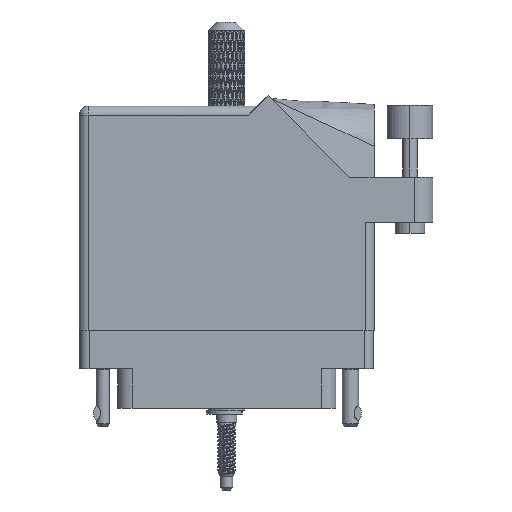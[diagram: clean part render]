
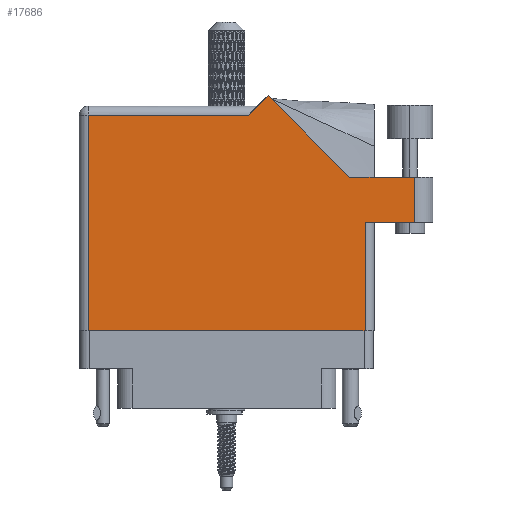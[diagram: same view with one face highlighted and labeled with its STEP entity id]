
A CAD part, front view. The second image highlights one B-rep face of the part: STEP entity #17686.
In plain terms, the highlighted face is planar.
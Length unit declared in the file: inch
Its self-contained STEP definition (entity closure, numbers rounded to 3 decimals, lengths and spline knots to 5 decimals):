
#356 = VERTEX_POINT ( 'NONE', #23343 ) ;
#3333 = VECTOR ( 'NONE', #69951, 39.37008 ) ;
#3750 = CARTESIAN_POINT ( 'NONE',  ( 1.217, 1.53, 0. ) ) ;
#3833 = ORIENTED_EDGE ( 'NONE', *, *, #64419, .T. ) ;
#4593 = ORIENTED_EDGE ( 'NONE', *, *, #90205, .T. ) ;
#4787 = VERTEX_POINT ( 'NONE', #7059 ) ;
#6399 = EDGE_CURVE ( 'NONE', #12704, #21247, #71066, .T. ) ;
#7059 = CARTESIAN_POINT ( 'NONE',  ( 2.285, 0.737, 0. ) ) ;
#7301 = EDGE_CURVE ( 'NONE', #24955, #42192, #51604, .T. ) ;
#7851 = VECTOR ( 'NONE', #73545, 39.37008 ) ;
#9972 = CARTESIAN_POINT ( 'NONE',  ( 0., 0., 0. ) ) ;
#11493 = CARTESIAN_POINT ( 'NONE',  ( 1.155, 1.468, 0. ) ) ;
#12704 = VERTEX_POINT ( 'NONE', #13270 ) ;
#13270 = CARTESIAN_POINT ( 'NONE',  ( 1.28771, 1.60071, 0. ) ) ;
#17686 = ADVANCED_FACE ( 'NONE', ( #64430 ), #88714, .F. ) ;
#21103 = DIRECTION ( 'NONE',  ( -0.707, -0.707, 0. ) ) ;
#21247 = VERTEX_POINT ( 'NONE', #11493 ) ;
#22135 = ORIENTED_EDGE ( 'NONE', *, *, #95997, .T. ) ;
#22268 = ORIENTED_EDGE ( 'NONE', *, *, #27672, .T. ) ;
#23196 = DIRECTION ( 'NONE',  ( -1., 0., 0. ) ) ;
#23343 = CARTESIAN_POINT ( 'NONE',  ( 1.84442, 1.044, 0. ) ) ;
#24955 = VERTEX_POINT ( 'NONE', #62414 ) ;
#27672 = EDGE_CURVE ( 'NONE', #356, #12704, #86226, .T. ) ;
#28164 = EDGE_LOOP ( 'NONE', ( #4593, #3833, #73130, #22268, #108743, #54055, #102697, #22135, #40379 ) ) ;
#31610 = LINE ( 'NONE', #111605, #92020 ) ;
#33352 = CARTESIAN_POINT ( 'NONE',  ( 0.062, 0., 0. ) ) ;
#36095 = CARTESIAN_POINT ( 'NONE',  ( 0., 1.53, 0. ) ) ;
#36884 = DIRECTION ( 'NONE',  ( 1., 0., 0. ) ) ;
#37159 = EDGE_CURVE ( 'NONE', #85621, #51917, #87926, .T. ) ;
#38554 = VERTEX_POINT ( 'NONE', #99038 ) ;
#40379 = ORIENTED_EDGE ( 'NONE', *, *, #7301, .T. ) ;
#42149 = DIRECTION ( 'NONE',  ( 0., -1., 0. ) ) ;
#42192 = VERTEX_POINT ( 'NONE', #77153 ) ;
#42554 = DIRECTION ( 'NONE',  ( -1., 0., 0. ) ) ;
#46876 = LINE ( 'NONE', #82608, #49634 ) ;
#49634 = VECTOR ( 'NONE', #42554, 39.37008 ) ;
#50713 = EDGE_CURVE ( 'NONE', #21247, #85621, #46876, .T. ) ;
#51604 = LINE ( 'NONE', #79600, #72307 ) ;
#51917 = VERTEX_POINT ( 'NONE', #102295 ) ;
#54055 = ORIENTED_EDGE ( 'NONE', *, *, #50713, .T. ) ;
#54512 = DIRECTION ( 'NONE',  ( 0., 0., -1. ) ) ;
#60694 = CARTESIAN_POINT ( 'NONE',  ( 2.285, 1.044, 0. ) ) ;
#62414 = CARTESIAN_POINT ( 'NONE',  ( 1.948, 0., 0. ) ) ;
#64419 = EDGE_CURVE ( 'NONE', #4787, #38554, #109209, .T. ) ;
#64430 = FACE_OUTER_BOUND ( 'NONE', #28164, .T. ) ;
#64701 = CARTESIAN_POINT ( 'NONE',  ( 1.84442, 1.044, 0. ) ) ;
#67826 = CARTESIAN_POINT ( 'NONE',  ( 2.41, 1.044, 0. ) ) ;
#69951 = DIRECTION ( 'NONE',  ( 0., 1., 0. ) ) ;
#70002 = LINE ( 'NONE', #67826, #101597 ) ;
#71066 = LINE ( 'NONE', #3750, #72522 ) ;
#72307 = VECTOR ( 'NONE', #88748, 39.37008 ) ;
#72522 = VECTOR ( 'NONE', #21103, 39.37008 ) ;
#73130 = ORIENTED_EDGE ( 'NONE', *, *, #83931, .T. ) ;
#73545 = DIRECTION ( 'NONE',  ( -0.707, 0.707, 0. ) ) ;
#77153 = CARTESIAN_POINT ( 'NONE',  ( 1.948, 0.737, 0. ) ) ;
#79600 = CARTESIAN_POINT ( 'NONE',  ( 1.948, 0.737, 0. ) ) ;
#80341 = DIRECTION ( 'NONE',  ( -1., 0., 0. ) ) ;
#82608 = CARTESIAN_POINT ( 'NONE',  ( 0., 1.468, 0. ) ) ;
#83931 = EDGE_CURVE ( 'NONE', #38554, #356, #70002, .T. ) ;
#85621 = VERTEX_POINT ( 'NONE', #97045 ) ;
#86226 = LINE ( 'NONE', #64701, #7851 ) ;
#87926 = LINE ( 'NONE', #33352, #96259 ) ;
#88714 = PLANE ( 'NONE',  #95332 ) ;
#88748 = DIRECTION ( 'NONE',  ( 0., 1., 0. ) ) ;
#89118 = LINE ( 'NONE', #9972, #96128 ) ;
#90205 = EDGE_CURVE ( 'NONE', #42192, #4787, #31610, .T. ) ;
#92020 = VECTOR ( 'NONE', #103111, 39.37008 ) ;
#95332 = AXIS2_PLACEMENT_3D ( 'NONE', #36095, #54512, #80341 ) ;
#95997 = EDGE_CURVE ( 'NONE', #51917, #24955, #89118, .T. ) ;
#96128 = VECTOR ( 'NONE', #36884, 39.37008 ) ;
#96259 = VECTOR ( 'NONE', #42149, 39.37008 ) ;
#97045 = CARTESIAN_POINT ( 'NONE',  ( 0.062, 1.468, 0. ) ) ;
#99038 = CARTESIAN_POINT ( 'NONE',  ( 2.285, 1.044, 0. ) ) ;
#101597 = VECTOR ( 'NONE', #23196, 39.37008 ) ;
#102295 = CARTESIAN_POINT ( 'NONE',  ( 0.062, 0., 0. ) ) ;
#102697 = ORIENTED_EDGE ( 'NONE', *, *, #37159, .T. ) ;
#103111 = DIRECTION ( 'NONE',  ( 1., 0., 0. ) ) ;
#108743 = ORIENTED_EDGE ( 'NONE', *, *, #6399, .T. ) ;
#109209 = LINE ( 'NONE', #60694, #3333 ) ;
#111605 = CARTESIAN_POINT ( 'NONE',  ( 2.01, 0.737, 0. ) ) ;
